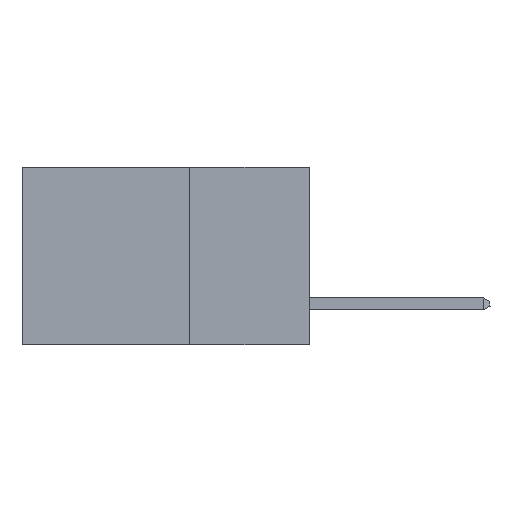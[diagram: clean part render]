
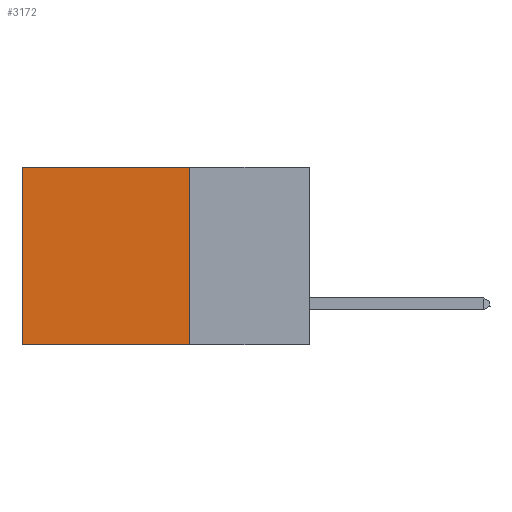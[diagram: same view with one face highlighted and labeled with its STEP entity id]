
A CAD part, left-side view. The second image highlights one B-rep face of the part: STEP entity #3172.
In plain terms, the highlighted planar face has unit normal (-1, 0, 0).
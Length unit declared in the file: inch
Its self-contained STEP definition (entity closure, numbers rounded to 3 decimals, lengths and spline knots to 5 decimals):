
#57 = ORIENTED_EDGE ( 'NONE', *, *, #18625, .F. ) ;
#68 = EDGE_CURVE ( 'NONE', #15503, #7747, #3493, .T. ) ;
#849 = LINE ( 'NONE', #17106, #12097 ) ;
#1555 = VERTEX_POINT ( 'NONE', #13485 ) ;
#2319 = EDGE_LOOP ( 'NONE', ( #14651, #57, #9105, #6211 ) ) ;
#3172 = ADVANCED_FACE ( 'NONE', ( #16015 ), #11341, .F. ) ;
#3493 = LINE ( 'NONE', #18549, #16342 ) ;
#3990 = DIRECTION ( 'NONE',  ( 0., 1., 0. ) ) ;
#5619 = DIRECTION ( 'NONE',  ( 0., 0., -1. ) ) ;
#5746 = CARTESIAN_POINT ( 'NONE',  ( 0.2875, 0.25, -0.37 ) ) ;
#6211 = ORIENTED_EDGE ( 'NONE', *, *, #10981, .T. ) ;
#6254 = VECTOR ( 'NONE', #3990, 39.37008 ) ;
#7747 = VERTEX_POINT ( 'NONE', #15111 ) ;
#8446 = DIRECTION ( 'NONE',  ( 0., 0., -1. ) ) ;
#8552 = LINE ( 'NONE', #11044, #12841 ) ;
#8598 = CARTESIAN_POINT ( 'NONE',  ( 0.2875, 0.25, -0.37 ) ) ;
#9064 = VERTEX_POINT ( 'NONE', #5746 ) ;
#9105 = ORIENTED_EDGE ( 'NONE', *, *, #12858, .F. ) ;
#9724 = DIRECTION ( 'NONE',  ( 1., 0., 0. ) ) ;
#10854 = DIRECTION ( 'NONE',  ( 0., 1., 0. ) ) ;
#10981 = EDGE_CURVE ( 'NONE', #1555, #15503, #8552, .T. ) ;
#11044 = CARTESIAN_POINT ( 'NONE',  ( 0.2875, 0.25, 0. ) ) ;
#11341 = PLANE ( 'NONE',  #16948 ) ;
#11613 = DIRECTION ( 'NONE',  ( 0., 0., -1. ) ) ;
#12097 = VECTOR ( 'NONE', #5619, 39.37008 ) ;
#12841 = VECTOR ( 'NONE', #10854, 39.37008 ) ;
#12858 = EDGE_CURVE ( 'NONE', #1555, #9064, #849, .T. ) ;
#13485 = CARTESIAN_POINT ( 'NONE',  ( 0.2875, 0.25, 0. ) ) ;
#14651 = ORIENTED_EDGE ( 'NONE', *, *, #68, .T. ) ;
#14760 = CARTESIAN_POINT ( 'NONE',  ( 0.2875, 0.6, 0. ) ) ;
#15111 = CARTESIAN_POINT ( 'NONE',  ( 0.2875, 0.6, -0.37 ) ) ;
#15503 = VERTEX_POINT ( 'NONE', #14760 ) ;
#16015 = FACE_OUTER_BOUND ( 'NONE', #2319, .T. ) ;
#16342 = VECTOR ( 'NONE', #11613, 39.37008 ) ;
#16948 = AXIS2_PLACEMENT_3D ( 'NONE', #17026, #9724, #8446 ) ;
#17026 = CARTESIAN_POINT ( 'NONE',  ( 0.2875, 0.25, 0. ) ) ;
#17106 = CARTESIAN_POINT ( 'NONE',  ( 0.2875, 0.25, 0. ) ) ;
#17996 = LINE ( 'NONE', #8598, #6254 ) ;
#18549 = CARTESIAN_POINT ( 'NONE',  ( 0.2875, 0.6, 0. ) ) ;
#18625 = EDGE_CURVE ( 'NONE', #9064, #7747, #17996, .T. ) ;
